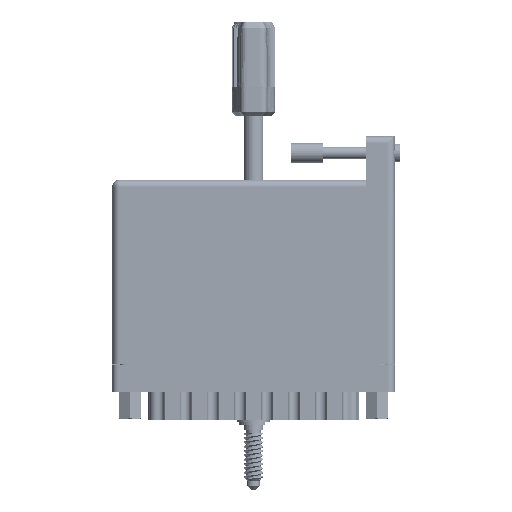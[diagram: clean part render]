
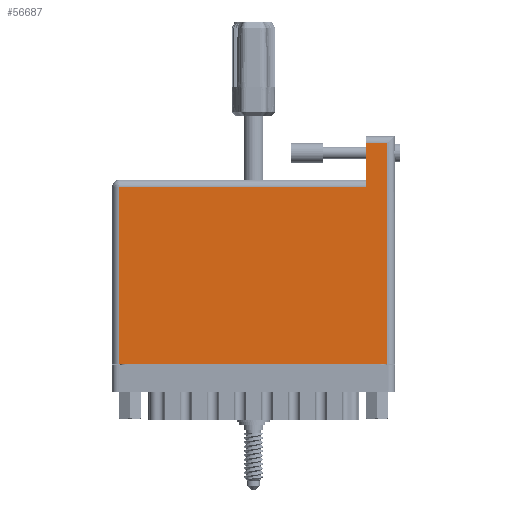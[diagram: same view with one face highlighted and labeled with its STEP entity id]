
A CAD part, front view. The second image highlights one B-rep face of the part: STEP entity #56687.
In plain terms, the highlighted face is planar.
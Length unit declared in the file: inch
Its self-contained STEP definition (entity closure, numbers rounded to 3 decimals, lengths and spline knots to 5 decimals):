
#74 = CARTESIAN_POINT ( 'NONE',  ( 0., 0., 0. ) ) ;
#231 = LINE ( 'NONE', #74, #58705 ) ;
#1362 = CARTESIAN_POINT ( 'NONE',  ( 2.438, 1.705, 0. ) ) ;
#3710 = CARTESIAN_POINT ( 'NONE',  ( 2.648, 0., 0. ) ) ;
#5965 = ORIENTED_EDGE ( 'NONE', *, *, #54352, .T. ) ;
#5971 = VECTOR ( 'NONE', #96870, 39.37008 ) ;
#7988 = DIRECTION ( 'NONE',  ( -1., 0., 0. ) ) ;
#13302 = VECTOR ( 'NONE', #39895, 39.37008 ) ;
#18734 = CARTESIAN_POINT ( 'NONE',  ( 0.07, 0., 0. ) ) ;
#19287 = CARTESIAN_POINT ( 'NONE',  ( 2.648, 2.195, 0. ) ) ;
#21334 = ORIENTED_EDGE ( 'NONE', *, *, #97215, .T. ) ;
#23864 = EDGE_LOOP ( 'NONE', ( #30848, #87322, #97290, #5965, #21334, #40031 ) ) ;
#27469 = VERTEX_POINT ( 'NONE', #49657 ) ;
#28870 = VECTOR ( 'NONE', #45462, 39.37008 ) ;
#30682 = CARTESIAN_POINT ( 'NONE',  ( 2.438, 2.195, 0. ) ) ;
#30848 = ORIENTED_EDGE ( 'NONE', *, *, #72301, .T. ) ;
#33608 = LINE ( 'NONE', #77599, #13302 ) ;
#36330 = CARTESIAN_POINT ( 'NONE',  ( 0.07, 0., 0. ) ) ;
#39895 = DIRECTION ( 'NONE',  ( -1., 0., 0. ) ) ;
#40031 = ORIENTED_EDGE ( 'NONE', *, *, #95947, .T. ) ;
#40957 = VECTOR ( 'NONE', #60965, 39.37008 ) ;
#42925 = CARTESIAN_POINT ( 'NONE',  ( 2.438, 2.125, 0. ) ) ;
#43001 = VERTEX_POINT ( 'NONE', #42925 ) ;
#43320 = DIRECTION ( 'NONE',  ( 0., -1., 0. ) ) ;
#45194 = CARTESIAN_POINT ( 'NONE',  ( 0.07, 1.705, 0. ) ) ;
#45462 = DIRECTION ( 'NONE',  ( -1., 0., 0. ) ) ;
#48201 = EDGE_CURVE ( 'NONE', #57821, #48593, #231, .T. ) ;
#48593 = VERTEX_POINT ( 'NONE', #3710 ) ;
#49657 = CARTESIAN_POINT ( 'NONE',  ( 2.648, 2.125, 0. ) ) ;
#51708 = VECTOR ( 'NONE', #43320, 39.37008 ) ;
#54352 = EDGE_CURVE ( 'NONE', #48593, #27469, #68054, .T. ) ;
#56687 = ADVANCED_FACE ( 'NONE', ( #62791 ), #76722, .F. ) ;
#57202 = AXIS2_PLACEMENT_3D ( 'NONE', #75765, #76086, #7988 ) ;
#57821 = VERTEX_POINT ( 'NONE', #18734 ) ;
#58705 = VECTOR ( 'NONE', #61431, 39.37008 ) ;
#58794 = EDGE_CURVE ( 'NONE', #82705, #57821, #61252, .T. ) ;
#60965 = DIRECTION ( 'NONE',  ( 0., -1., 0. ) ) ;
#61252 = LINE ( 'NONE', #36330, #51708 ) ;
#61431 = DIRECTION ( 'NONE',  ( 1., 0., 0. ) ) ;
#62464 = LINE ( 'NONE', #30682, #40957 ) ;
#62791 = FACE_OUTER_BOUND ( 'NONE', #23864, .T. ) ;
#68054 = LINE ( 'NONE', #19287, #5971 ) ;
#72301 = EDGE_CURVE ( 'NONE', #73612, #82705, #33608, .T. ) ;
#73612 = VERTEX_POINT ( 'NONE', #1362 ) ;
#75765 = CARTESIAN_POINT ( 'NONE',  ( 0., 1.775, 0. ) ) ;
#76086 = DIRECTION ( 'NONE',  ( 0., 0., -1. ) ) ;
#76722 = PLANE ( 'NONE',  #57202 ) ;
#77599 = CARTESIAN_POINT ( 'NONE',  ( 0., 1.705, 0. ) ) ;
#82705 = VERTEX_POINT ( 'NONE', #45194 ) ;
#87322 = ORIENTED_EDGE ( 'NONE', *, *, #58794, .T. ) ;
#89646 = LINE ( 'NONE', #91735, #28870 ) ;
#91735 = CARTESIAN_POINT ( 'NONE',  ( 0., 2.125, 0. ) ) ;
#95947 = EDGE_CURVE ( 'NONE', #43001, #73612, #62464, .T. ) ;
#96870 = DIRECTION ( 'NONE',  ( 0., 1., 0. ) ) ;
#97215 = EDGE_CURVE ( 'NONE', #27469, #43001, #89646, .T. ) ;
#97290 = ORIENTED_EDGE ( 'NONE', *, *, #48201, .T. ) ;
